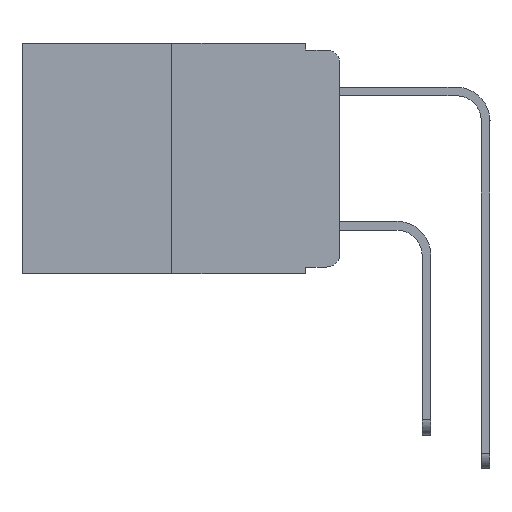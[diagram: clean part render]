
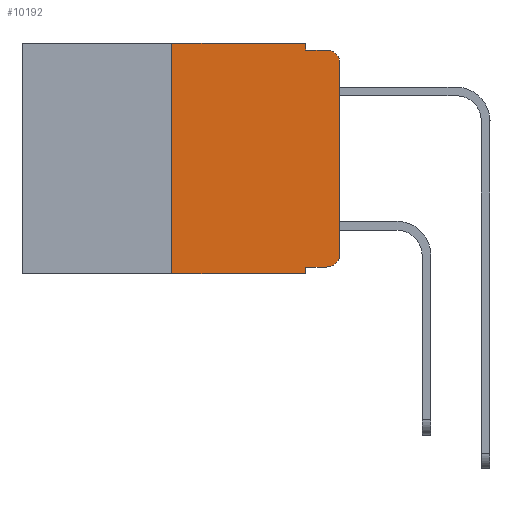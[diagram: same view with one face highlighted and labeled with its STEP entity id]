
A CAD part, left-side view. The second image highlights one B-rep face of the part: STEP entity #10192.
In plain terms, the highlighted planar face has unit normal (-1, 0, 0).
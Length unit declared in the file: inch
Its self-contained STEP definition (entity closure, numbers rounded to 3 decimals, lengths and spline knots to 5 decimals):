
#42 = VERTEX_POINT ( 'NONE', #5617 ) ;
#720 = VERTEX_POINT ( 'NONE', #23218 ) ;
#1070 = VERTEX_POINT ( 'NONE', #24463 ) ;
#1784 = DIRECTION ( 'NONE',  ( 0., 0., -1. ) ) ;
#2180 = EDGE_CURVE ( 'NONE', #19084, #14682, #7061, .T. ) ;
#2458 = EDGE_LOOP ( 'NONE', ( #20818, #20443, #23502, #20745, #15410, #17778, #3667, #5071, #13700, #9078 ) ) ;
#3034 = DIRECTION ( 'NONE',  ( 0., -1., 0. ) ) ;
#3107 = VECTOR ( 'NONE', #9199, 39.37008 ) ;
#3274 = LINE ( 'NONE', #16243, #25567 ) ;
#3667 = ORIENTED_EDGE ( 'NONE', *, *, #5608, .T. ) ;
#3686 = EDGE_CURVE ( 'NONE', #14682, #27264, #14871, .T. ) ;
#4363 = CARTESIAN_POINT ( 'NONE',  ( 0., 0.02, -0.01 ) ) ;
#5071 = ORIENTED_EDGE ( 'NONE', *, *, #23123, .F. ) ;
#5102 = CARTESIAN_POINT ( 'NONE',  ( 0., 0.02, -0.313 ) ) ;
#5206 = EDGE_CURVE ( 'NONE', #14825, #27264, #22724, .T. ) ;
#5608 = EDGE_CURVE ( 'NONE', #26446, #12966, #3274, .T. ) ;
#5617 = CARTESIAN_POINT ( 'NONE',  ( 0., 0.25, 0. ) ) ;
#5880 = CARTESIAN_POINT ( 'NONE',  ( 0., 0.051, 0. ) ) ;
#6403 = EDGE_CURVE ( 'NONE', #42, #19084, #18958, .T. ) ;
#7061 = LINE ( 'NONE', #19436, #23504 ) ;
#7404 = DIRECTION ( 'NONE',  ( 0., 0., -1. ) ) ;
#7966 = DIRECTION ( 'NONE',  ( 0., -1., 0. ) ) ;
#8715 = CARTESIAN_POINT ( 'NONE',  ( 0., 0.02, -0.333 ) ) ;
#9078 = ORIENTED_EDGE ( 'NONE', *, *, #13184, .T. ) ;
#9199 = DIRECTION ( 'NONE',  ( 0., -1., 0. ) ) ;
#9749 = EDGE_CURVE ( 'NONE', #720, #14825, #27033, .T. ) ;
#9905 = DIRECTION ( 'NONE',  ( 0., 0., 1. ) ) ;
#10105 = CARTESIAN_POINT ( 'NONE',  ( 0., 0.473, 0. ) ) ;
#10192 = ADVANCED_FACE ( 'NONE', ( #22734 ), #25083, .F. ) ;
#10273 = CARTESIAN_POINT ( 'NONE',  ( 0., 0.473, 0. ) ) ;
#10501 = AXIS2_PLACEMENT_3D ( 'NONE', #5102, #20285, #7404 ) ;
#10525 = VECTOR ( 'NONE', #11427, 39.37008 ) ;
#10848 = CARTESIAN_POINT ( 'NONE',  ( 0., 0., 0. ) ) ;
#11035 = VECTOR ( 'NONE', #9905, 39.37008 ) ;
#11427 = DIRECTION ( 'NONE',  ( 0., -1., 0. ) ) ;
#11441 = VECTOR ( 'NONE', #17647, 39.37008 ) ;
#12125 = LINE ( 'NONE', #15524, #11441 ) ;
#12430 = DIRECTION ( 'NONE',  ( 1., 0., 0. ) ) ;
#12966 = VERTEX_POINT ( 'NONE', #21684 ) ;
#13184 = EDGE_CURVE ( 'NONE', #17996, #720, #17571, .T. ) ;
#13560 = CARTESIAN_POINT ( 'NONE',  ( 0., 0.051, -0.01 ) ) ;
#13700 = ORIENTED_EDGE ( 'NONE', *, *, #21707, .T. ) ;
#14682 = VERTEX_POINT ( 'NONE', #27770 ) ;
#14825 = VERTEX_POINT ( 'NONE', #19762 ) ;
#14871 = LINE ( 'NONE', #13560, #3107 ) ;
#14895 = LINE ( 'NONE', #26228, #10525 ) ;
#15048 = DIRECTION ( 'NONE',  ( -1., 0., 0. ) ) ;
#15208 = DIRECTION ( 'NONE',  ( 0., 0., -1. ) ) ;
#15410 = ORIENTED_EDGE ( 'NONE', *, *, #6403, .F. ) ;
#15524 = CARTESIAN_POINT ( 'NONE',  ( 0., 0.051, 0. ) ) ;
#16243 = CARTESIAN_POINT ( 'NONE',  ( 0., 0.473, -0.343 ) ) ;
#16719 = CARTESIAN_POINT ( 'NONE',  ( 0., 0.25, -0.343 ) ) ;
#17571 = CIRCLE ( 'NONE', #10501, 0.02 ) ;
#17647 = DIRECTION ( 'NONE',  ( 0., 0., -1. ) ) ;
#17778 = ORIENTED_EDGE ( 'NONE', *, *, #24504, .F. ) ;
#17996 = VERTEX_POINT ( 'NONE', #8715 ) ;
#18293 = VECTOR ( 'NONE', #7966, 39.37008 ) ;
#18958 = LINE ( 'NONE', #10105, #18293 ) ;
#19084 = VERTEX_POINT ( 'NONE', #5880 ) ;
#19436 = CARTESIAN_POINT ( 'NONE',  ( 0., 0.051, 0. ) ) ;
#19762 = CARTESIAN_POINT ( 'NONE',  ( 0., 0., -0.03 ) ) ;
#20285 = DIRECTION ( 'NONE',  ( -1., 0., 0. ) ) ;
#20443 = ORIENTED_EDGE ( 'NONE', *, *, #5206, .T. ) ;
#20745 = ORIENTED_EDGE ( 'NONE', *, *, #2180, .F. ) ;
#20818 = ORIENTED_EDGE ( 'NONE', *, *, #9749, .T. ) ;
#21443 = VECTOR ( 'NONE', #27782, 39.37008 ) ;
#21684 = CARTESIAN_POINT ( 'NONE',  ( 0., 0.051, -0.343 ) ) ;
#21707 = EDGE_CURVE ( 'NONE', #1070, #17996, #14895, .T. ) ;
#22724 = CIRCLE ( 'NONE', #22993, 0.02 ) ;
#22734 = FACE_OUTER_BOUND ( 'NONE', #2458, .T. ) ;
#22993 = AXIS2_PLACEMENT_3D ( 'NONE', #27656, #15048, #1784 ) ;
#23123 = EDGE_CURVE ( 'NONE', #1070, #12966, #12125, .T. ) ;
#23218 = CARTESIAN_POINT ( 'NONE',  ( 0., 0., -0.313 ) ) ;
#23502 = ORIENTED_EDGE ( 'NONE', *, *, #3686, .F. ) ;
#23504 = VECTOR ( 'NONE', #15208, 39.37008 ) ;
#24463 = CARTESIAN_POINT ( 'NONE',  ( 0., 0.051, -0.333 ) ) ;
#24504 = EDGE_CURVE ( 'NONE', #26446, #42, #27273, .T. ) ;
#25083 = PLANE ( 'NONE',  #27652 ) ;
#25567 = VECTOR ( 'NONE', #3034, 39.37008 ) ;
#26228 = CARTESIAN_POINT ( 'NONE',  ( 0., 0.051, -0.333 ) ) ;
#26446 = VERTEX_POINT ( 'NONE', #16719 ) ;
#26779 = CARTESIAN_POINT ( 'NONE',  ( 0., 0.25, 0. ) ) ;
#27033 = LINE ( 'NONE', #10848, #21443 ) ;
#27219 = DIRECTION ( 'NONE',  ( 0., 0., -1. ) ) ;
#27264 = VERTEX_POINT ( 'NONE', #4363 ) ;
#27273 = LINE ( 'NONE', #26779, #11035 ) ;
#27652 = AXIS2_PLACEMENT_3D ( 'NONE', #10273, #12430, #27219 ) ;
#27656 = CARTESIAN_POINT ( 'NONE',  ( 0., 0.02, -0.03 ) ) ;
#27770 = CARTESIAN_POINT ( 'NONE',  ( 0., 0.051, -0.01 ) ) ;
#27782 = DIRECTION ( 'NONE',  ( 0., 0., 1. ) ) ;
